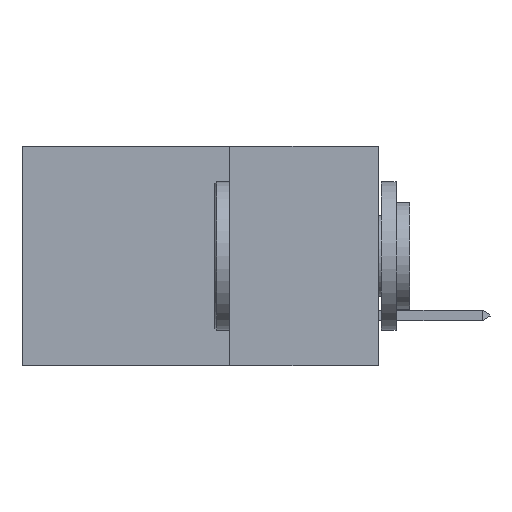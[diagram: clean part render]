
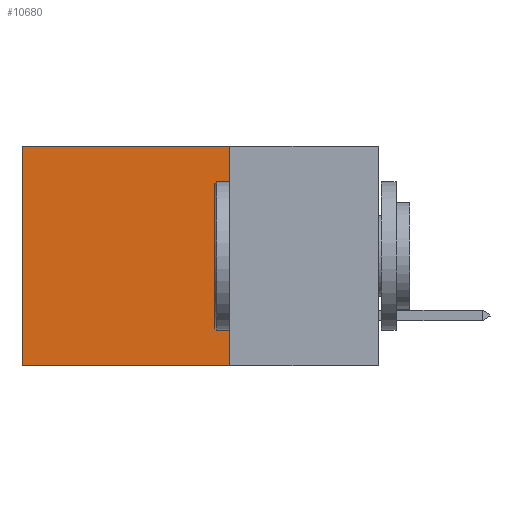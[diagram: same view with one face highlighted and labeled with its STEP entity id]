
A CAD part, left-side view. The second image highlights one B-rep face of the part: STEP entity #10680.
In plain terms, the highlighted planar face has unit normal (-1, 0, 0).
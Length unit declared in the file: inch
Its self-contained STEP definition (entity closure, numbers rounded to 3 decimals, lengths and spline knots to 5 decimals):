
#217 = ORIENTED_EDGE ( 'NONE', *, *, #8037, .T. ) ;
#270 = DIRECTION ( 'NONE',  ( 0., 1., 0. ) ) ;
#810 = VERTEX_POINT ( 'NONE', #8109 ) ;
#889 = FACE_OUTER_BOUND ( 'NONE', #7738, .T. ) ;
#1336 = EDGE_CURVE ( 'NONE', #810, #6984, #8018, .T. ) ;
#1788 = CARTESIAN_POINT ( 'NONE',  ( 0.298, 0.25, 0. ) ) ;
#2650 = CARTESIAN_POINT ( 'NONE',  ( 0.298, 0.6, 0. ) ) ;
#3789 = CARTESIAN_POINT ( 'NONE',  ( 0.298, 0.6, 0. ) ) ;
#5689 = DIRECTION ( 'NONE',  ( 1., 0., 0. ) ) ;
#6165 = LINE ( 'NONE', #12257, #10574 ) ;
#6923 = ORIENTED_EDGE ( 'NONE', *, *, #13332, .F. ) ;
#6984 = VERTEX_POINT ( 'NONE', #8734 ) ;
#7178 = AXIS2_PLACEMENT_3D ( 'NONE', #9818, #5689, #12987 ) ;
#7738 = EDGE_LOOP ( 'NONE', ( #217, #6923, #12765, #8967 ) ) ;
#7772 = PLANE ( 'NONE',  #7178 ) ;
#7941 = VERTEX_POINT ( 'NONE', #2650 ) ;
#8018 = LINE ( 'NONE', #1788, #10428 ) ;
#8037 = EDGE_CURVE ( 'NONE', #7941, #12784, #13242, .T. ) ;
#8109 = CARTESIAN_POINT ( 'NONE',  ( 0.298, 0.25, 0. ) ) ;
#8734 = CARTESIAN_POINT ( 'NONE',  ( 0.298, 0.25, -0.37 ) ) ;
#8967 = ORIENTED_EDGE ( 'NONE', *, *, #9654, .T. ) ;
#9654 = EDGE_CURVE ( 'NONE', #810, #7941, #6165, .T. ) ;
#9780 = VECTOR ( 'NONE', #13358, 39.37008 ) ;
#9818 = CARTESIAN_POINT ( 'NONE',  ( 0.298, 0.25, 0. ) ) ;
#9979 = DIRECTION ( 'NONE',  ( 0., 0., -1. ) ) ;
#10168 = DIRECTION ( 'NONE',  ( 0., 1., 0. ) ) ;
#10186 = VECTOR ( 'NONE', #270, 39.37008 ) ;
#10428 = VECTOR ( 'NONE', #9979, 39.37008 ) ;
#10574 = VECTOR ( 'NONE', #10168, 39.37008 ) ;
#10680 = ADVANCED_FACE ( 'NONE', ( #889 ), #7772, .F. ) ;
#10825 = CARTESIAN_POINT ( 'NONE',  ( 0.298, 0.6, -0.37 ) ) ;
#12257 = CARTESIAN_POINT ( 'NONE',  ( 0.298, 0.25, 0. ) ) ;
#12765 = ORIENTED_EDGE ( 'NONE', *, *, #1336, .F. ) ;
#12784 = VERTEX_POINT ( 'NONE', #10825 ) ;
#12987 = DIRECTION ( 'NONE',  ( 0., 0., -1. ) ) ;
#13014 = CARTESIAN_POINT ( 'NONE',  ( 0.298, 0.25, -0.37 ) ) ;
#13242 = LINE ( 'NONE', #3789, #9780 ) ;
#13332 = EDGE_CURVE ( 'NONE', #6984, #12784, #13488, .T. ) ;
#13358 = DIRECTION ( 'NONE',  ( 0., 0., -1. ) ) ;
#13488 = LINE ( 'NONE', #13014, #10186 ) ;
